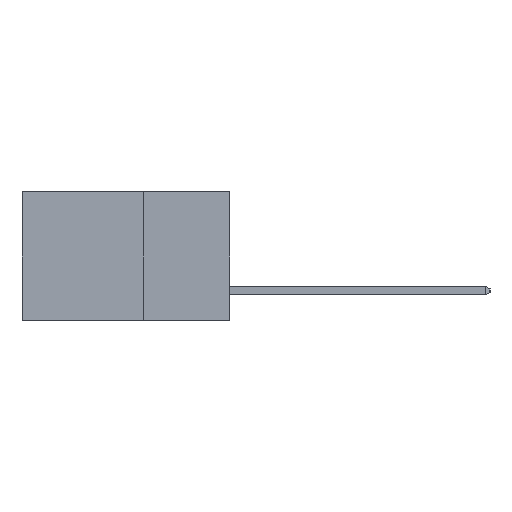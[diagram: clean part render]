
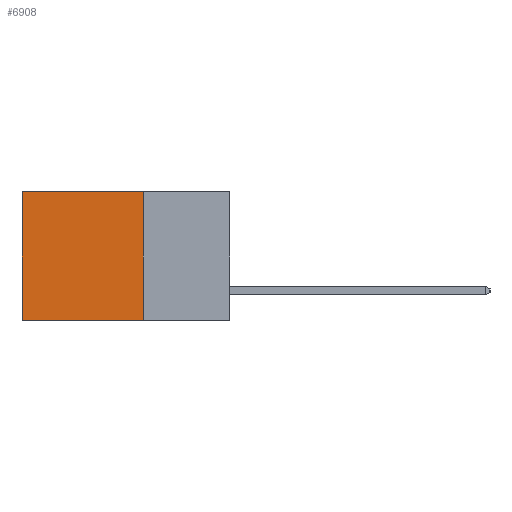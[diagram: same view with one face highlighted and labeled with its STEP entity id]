
A CAD part, left-side view. The second image highlights one B-rep face of the part: STEP entity #6908.
In plain terms, the highlighted planar face has unit normal (-1, 0, 0).
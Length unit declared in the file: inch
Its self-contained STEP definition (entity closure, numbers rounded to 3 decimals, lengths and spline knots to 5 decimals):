
#455 = ORIENTED_EDGE ( 'NONE', *, *, #3656, .T. ) ;
#2446 = EDGE_CURVE ( 'NONE', #14057, #9169, #6584, .T. ) ;
#2776 = VECTOR ( 'NONE', #3784, 39.37008 ) ;
#2835 = LINE ( 'NONE', #16439, #9927 ) ;
#2966 = AXIS2_PLACEMENT_3D ( 'NONE', #12937, #4566, #14314 ) ;
#3656 = EDGE_CURVE ( 'NONE', #17286, #8042, #17819, .T. ) ;
#3724 = CARTESIAN_POINT ( 'NONE',  ( 0.2615, 0.25, -0.37 ) ) ;
#3748 = DIRECTION ( 'NONE',  ( 0., 0., -1. ) ) ;
#3784 = DIRECTION ( 'NONE',  ( 0., 1., 0. ) ) ;
#4245 = VECTOR ( 'NONE', #3748, 39.37008 ) ;
#4566 = DIRECTION ( 'NONE',  ( 1., 0., 0. ) ) ;
#4704 = CARTESIAN_POINT ( 'NONE',  ( 0.2615, 0.25, -0.37 ) ) ;
#5126 = ORIENTED_EDGE ( 'NONE', *, *, #17580, .T. ) ;
#5703 = EDGE_CURVE ( 'NONE', #17286, #14057, #14935, .T. ) ;
#5871 = VECTOR ( 'NONE', #8172, 39.37008 ) ;
#6584 = LINE ( 'NONE', #4704, #2776 ) ;
#6908 = ADVANCED_FACE ( 'NONE', ( #10344 ), #15632, .F. ) ;
#8042 = VERTEX_POINT ( 'NONE', #16743 ) ;
#8172 = DIRECTION ( 'NONE',  ( 0., 1., 0. ) ) ;
#8355 = CARTESIAN_POINT ( 'NONE',  ( 0.2615, 0.25, 0. ) ) ;
#9169 = VERTEX_POINT ( 'NONE', #17975 ) ;
#9927 = VECTOR ( 'NONE', #17841, 39.37008 ) ;
#10073 = EDGE_LOOP ( 'NONE', ( #5126, #13039, #11211, #455 ) ) ;
#10344 = FACE_OUTER_BOUND ( 'NONE', #10073, .T. ) ;
#11211 = ORIENTED_EDGE ( 'NONE', *, *, #5703, .F. ) ;
#12937 = CARTESIAN_POINT ( 'NONE',  ( 0.2615, 0.25, -0.37 ) ) ;
#13039 = ORIENTED_EDGE ( 'NONE', *, *, #2446, .F. ) ;
#13256 = CARTESIAN_POINT ( 'NONE',  ( 0.2615, 0.25, -0.37 ) ) ;
#14057 = VERTEX_POINT ( 'NONE', #13256 ) ;
#14314 = DIRECTION ( 'NONE',  ( 0., 0., -1. ) ) ;
#14468 = CARTESIAN_POINT ( 'NONE',  ( 0.2615, 0.25, 0. ) ) ;
#14935 = LINE ( 'NONE', #3724, #4245 ) ;
#15632 = PLANE ( 'NONE',  #2966 ) ;
#16439 = CARTESIAN_POINT ( 'NONE',  ( 0.2615, 0.6, -0.37 ) ) ;
#16743 = CARTESIAN_POINT ( 'NONE',  ( 0.2615, 0.6, 0. ) ) ;
#17286 = VERTEX_POINT ( 'NONE', #14468 ) ;
#17580 = EDGE_CURVE ( 'NONE', #8042, #9169, #2835, .T. ) ;
#17819 = LINE ( 'NONE', #8355, #5871 ) ;
#17841 = DIRECTION ( 'NONE',  ( 0., 0., -1. ) ) ;
#17975 = CARTESIAN_POINT ( 'NONE',  ( 0.2615, 0.6, -0.37 ) ) ;
